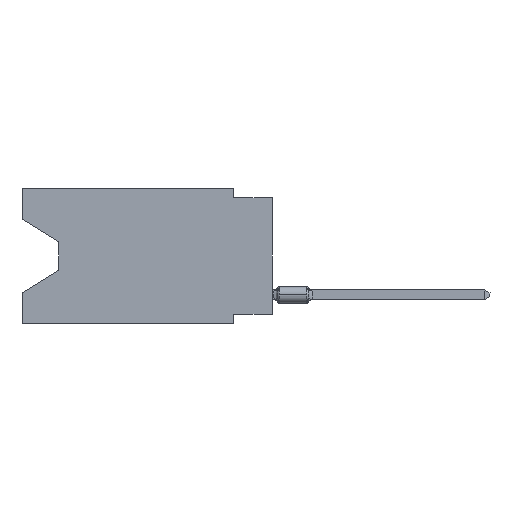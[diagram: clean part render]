
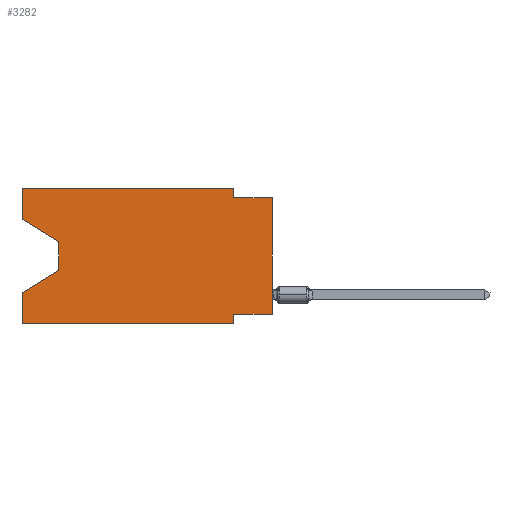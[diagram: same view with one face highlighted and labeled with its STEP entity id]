
A CAD part, left-side view. The second image highlights one B-rep face of the part: STEP entity #3282.
In plain terms, the highlighted planar face has unit normal (-1, 0, 0).
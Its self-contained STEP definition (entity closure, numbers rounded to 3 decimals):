
#99 = EDGE_CURVE ( 'NONE', #4230, #27353, #27637, .T. ) ;
#264 = CARTESIAN_POINT ( 'NONE',  ( 0., 13.97, -5.385 ) ) ;
#645 = EDGE_CURVE ( 'NONE', #24028, #809, #22854, .T. ) ;
#731 = ORIENTED_EDGE ( 'NONE', *, *, #23314, .F. ) ;
#809 = VERTEX_POINT ( 'NONE', #2110 ) ;
#2110 = CARTESIAN_POINT ( 'NONE',  ( 0., 2.54, -8.89 ) ) ;
#2158 = VERTEX_POINT ( 'NONE', #25902 ) ;
#2205 = DIRECTION ( 'NONE',  ( 0., -1., 0. ) ) ;
#2469 = VECTOR ( 'NONE', #7804, 1000. ) ;
#2524 = VECTOR ( 'NONE', #23329, 1000. ) ;
#3030 = LINE ( 'NONE', #18145, #9563 ) ;
#3106 = DIRECTION ( 'NONE',  ( 0., -1., 0. ) ) ;
#3282 = ADVANCED_FACE ( 'NONE', ( #8274 ), #27895, .F. ) ;
#3477 = EDGE_CURVE ( 'NONE', #6014, #6452, #30596, .T. ) ;
#3527 = VECTOR ( 'NONE', #26006, 1000. ) ;
#4230 = VERTEX_POINT ( 'NONE', #13039 ) ;
#4732 = LINE ( 'NONE', #21329, #29195 ) ;
#5106 = CARTESIAN_POINT ( 'NONE',  ( 0., 2.54, 0. ) ) ;
#5496 = ORIENTED_EDGE ( 'NONE', *, *, #21175, .F. ) ;
#5786 = VERTEX_POINT ( 'NONE', #264 ) ;
#5890 = DIRECTION ( 'NONE',  ( 0., 0., -1. ) ) ;
#6014 = VERTEX_POINT ( 'NONE', #5106 ) ;
#6198 = VERTEX_POINT ( 'NONE', #13572 ) ;
#6452 = VERTEX_POINT ( 'NONE', #14981 ) ;
#7573 = ORIENTED_EDGE ( 'NONE', *, *, #99, .T. ) ;
#7725 = CARTESIAN_POINT ( 'NONE',  ( 0., 0., 0. ) ) ;
#7804 = DIRECTION ( 'NONE',  ( 0., 0., 1. ) ) ;
#8035 = LINE ( 'NONE', #30031, #29367 ) ;
#8054 = AXIS2_PLACEMENT_3D ( 'NONE', #10837, #15920, #5890 ) ;
#8274 = FACE_OUTER_BOUND ( 'NONE', #23080, .T. ) ;
#8403 = CARTESIAN_POINT ( 'NONE',  ( 0., 13.97, -3.505 ) ) ;
#8669 = EDGE_CURVE ( 'NONE', #2158, #6198, #4732, .T. ) ;
#8743 = CARTESIAN_POINT ( 'NONE',  ( 0., 2.54, 0. ) ) ;
#9563 = VECTOR ( 'NONE', #20536, 1000. ) ;
#9776 = DIRECTION ( 'NONE',  ( 0., 0., -1. ) ) ;
#9858 = DIRECTION ( 'NONE',  ( 0., 0.855, -0.519 ) ) ;
#10400 = LINE ( 'NONE', #29849, #26784 ) ;
#10689 = EDGE_CURVE ( 'NONE', #5786, #22973, #14644, .T. ) ;
#10837 = CARTESIAN_POINT ( 'NONE',  ( 0., 16.383, 0. ) ) ;
#11157 = VECTOR ( 'NONE', #12588, 1000. ) ;
#11829 = VERTEX_POINT ( 'NONE', #12784 ) ;
#12127 = LINE ( 'NONE', #29338, #2469 ) ;
#12588 = DIRECTION ( 'NONE',  ( 0., 1., 0. ) ) ;
#12734 = ORIENTED_EDGE ( 'NONE', *, *, #8669, .F. ) ;
#12784 = CARTESIAN_POINT ( 'NONE',  ( 0., 2.54, -8.255 ) ) ;
#13039 = CARTESIAN_POINT ( 'NONE',  ( 0., 0., -8.255 ) ) ;
#13572 = CARTESIAN_POINT ( 'NONE',  ( 0., 16.383, 0. ) ) ;
#13737 = CARTESIAN_POINT ( 'NONE',  ( 0., 16.383, -8.89 ) ) ;
#13954 = ORIENTED_EDGE ( 'NONE', *, *, #645, .T. ) ;
#14644 = LINE ( 'NONE', #22147, #21671 ) ;
#14981 = CARTESIAN_POINT ( 'NONE',  ( 0., 2.54, -0.635 ) ) ;
#15423 = ORIENTED_EDGE ( 'NONE', *, *, #20516, .F. ) ;
#15920 = DIRECTION ( 'NONE',  ( 1., 0., 0. ) ) ;
#16306 = ORIENTED_EDGE ( 'NONE', *, *, #18048, .F. ) ;
#16615 = ORIENTED_EDGE ( 'NONE', *, *, #3477, .F. ) ;
#16752 = VECTOR ( 'NONE', #17762, 1000. ) ;
#17192 = VECTOR ( 'NONE', #2205, 1000. ) ;
#17256 = VECTOR ( 'NONE', #25822, 1000. ) ;
#17762 = DIRECTION ( 'NONE',  ( 0., 0., 1. ) ) ;
#18048 = EDGE_CURVE ( 'NONE', #24028, #22973, #12127, .T. ) ;
#18145 = CARTESIAN_POINT ( 'NONE',  ( 0., 2.54, -8.89 ) ) ;
#18274 = LINE ( 'NONE', #25756, #11157 ) ;
#18411 = ORIENTED_EDGE ( 'NONE', *, *, #24851, .F. ) ;
#20026 = CARTESIAN_POINT ( 'NONE',  ( 0., 16.383, -6.852 ) ) ;
#20516 = EDGE_CURVE ( 'NONE', #6198, #6014, #8035, .T. ) ;
#20536 = DIRECTION ( 'NONE',  ( 0., 0., -1. ) ) ;
#21047 = LINE ( 'NONE', #30756, #3527 ) ;
#21175 = EDGE_CURVE ( 'NONE', #6452, #27353, #24204, .T. ) ;
#21329 = CARTESIAN_POINT ( 'NONE',  ( 0., 16.383, 0. ) ) ;
#21671 = VECTOR ( 'NONE', #9858, 1000. ) ;
#22147 = CARTESIAN_POINT ( 'NONE',  ( 0., 13.97, -5.385 ) ) ;
#22854 = LINE ( 'NONE', #13737, #2524 ) ;
#22937 = CARTESIAN_POINT ( 'NONE',  ( 0., 0., -0.635 ) ) ;
#22973 = VERTEX_POINT ( 'NONE', #20026 ) ;
#23080 = EDGE_LOOP ( 'NONE', ( #28474, #25459, #25497, #16306, #13954, #731, #18411, #7573, #5496, #16615, #15423, #12734 ) ) ;
#23209 = VERTEX_POINT ( 'NONE', #8403 ) ;
#23314 = EDGE_CURVE ( 'NONE', #11829, #809, #3030, .T. ) ;
#23329 = DIRECTION ( 'NONE',  ( 0., -1., 0. ) ) ;
#24028 = VERTEX_POINT ( 'NONE', #24940 ) ;
#24204 = LINE ( 'NONE', #24529, #17192 ) ;
#24529 = CARTESIAN_POINT ( 'NONE',  ( 0., 0., -0.635 ) ) ;
#24591 = EDGE_CURVE ( 'NONE', #2158, #23209, #21047, .T. ) ;
#24851 = EDGE_CURVE ( 'NONE', #4230, #11829, #18274, .T. ) ;
#24940 = CARTESIAN_POINT ( 'NONE',  ( 0., 16.383, -8.89 ) ) ;
#25459 = ORIENTED_EDGE ( 'NONE', *, *, #26003, .T. ) ;
#25497 = ORIENTED_EDGE ( 'NONE', *, *, #10689, .T. ) ;
#25756 = CARTESIAN_POINT ( 'NONE',  ( 0., 0., -8.255 ) ) ;
#25822 = DIRECTION ( 'NONE',  ( 0., 0., -1. ) ) ;
#25902 = CARTESIAN_POINT ( 'NONE',  ( 0., 16.383, -2.038 ) ) ;
#26003 = EDGE_CURVE ( 'NONE', #23209, #5786, #10400, .T. ) ;
#26006 = DIRECTION ( 'NONE',  ( 0., -0.855, -0.519 ) ) ;
#26427 = DIRECTION ( 'NONE',  ( 0., 0., 1. ) ) ;
#26784 = VECTOR ( 'NONE', #9776, 1000. ) ;
#27353 = VERTEX_POINT ( 'NONE', #22937 ) ;
#27637 = LINE ( 'NONE', #7725, #16752 ) ;
#27895 = PLANE ( 'NONE',  #8054 ) ;
#28474 = ORIENTED_EDGE ( 'NONE', *, *, #24591, .T. ) ;
#29195 = VECTOR ( 'NONE', #26427, 1000. ) ;
#29338 = CARTESIAN_POINT ( 'NONE',  ( 0., 16.383, 0. ) ) ;
#29367 = VECTOR ( 'NONE', #3106, 1000. ) ;
#29849 = CARTESIAN_POINT ( 'NONE',  ( 0., 13.97, -3.505 ) ) ;
#30031 = CARTESIAN_POINT ( 'NONE',  ( 0., 16.383, 0. ) ) ;
#30596 = LINE ( 'NONE', #8743, #17256 ) ;
#30756 = CARTESIAN_POINT ( 'NONE',  ( 0., 16.383, -2.038 ) ) ;
